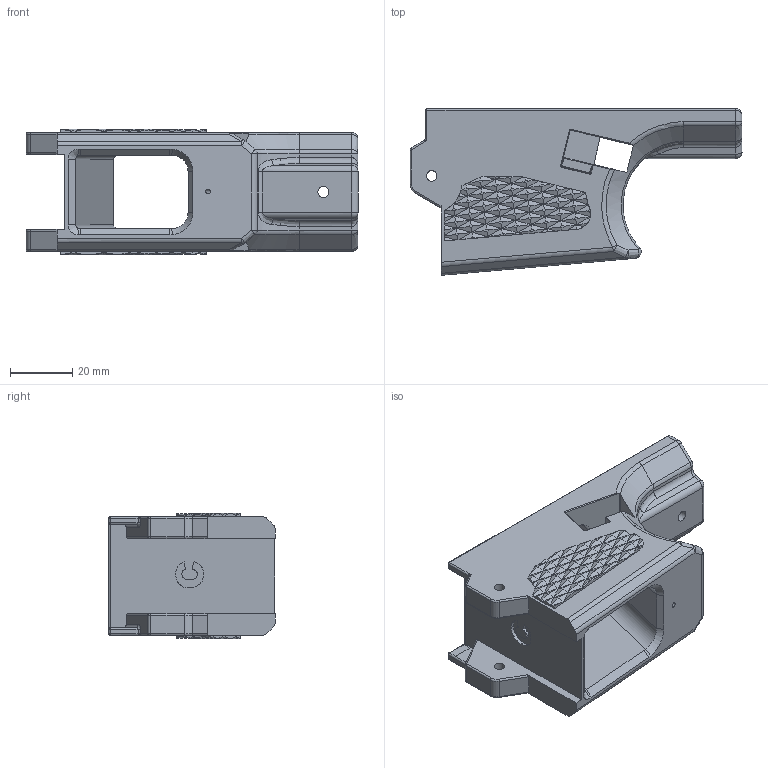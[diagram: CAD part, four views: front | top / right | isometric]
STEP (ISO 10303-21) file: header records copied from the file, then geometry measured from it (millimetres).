
FILE_DESCRIPTION(/* description */ (''),/* implementation_level */ '2;1');
FILE_NAME(/* author */ (''),/* organization */ (''),/* preprocessor_version */ 'ST-DEVELOPER v15.2',/* originating_system */ 'Autodesk Translator Framework v2.0.0.5431',/* authorisation */ '');
FILE_SCHEMA (('AUTOMOTIVE_DESIGN { 1 0 10303 214 3 1 1 }'));
Length unit declared in the file: centimetre
Products named in the file (1): MOD9 v3X Final Version C
Bounding box: 106.31 x 53.3 x 40.34 mm (x, y, z)
Volume: 81537.5 mm3; surface area: 24993.9 mm2
Topology: 1 solids, 1 shells, 767 faces, 1803 edges, 1030 vertices
Faces by surface type: plane 549, cylinder 91, bspline 90, sphere 16, torus 13, cone 8
Full cylindrical faces by diameter (mm): 1.5 x1, 3.4 x2, 3.5 x1, 4 x1
Entity records: 22936 total; most frequent: CARTESIAN_POINT 6033, ORIENTED_EDGE 3578, DIRECTION 3274, EDGE_CURVE 1789, LINE 1370, VECTOR 1370, VERTEX_POINT 1030, AXIS2_PLACEMENT_3D 952
